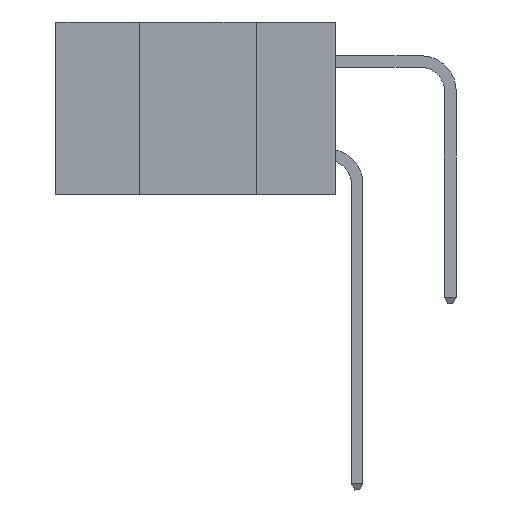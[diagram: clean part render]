
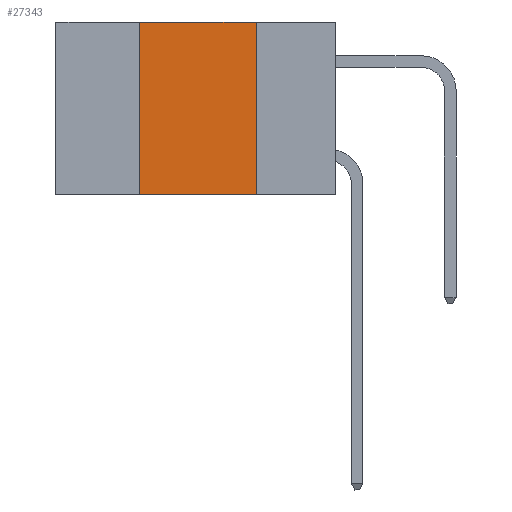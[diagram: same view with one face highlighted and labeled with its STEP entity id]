
A CAD part, left-side view. The second image highlights one B-rep face of the part: STEP entity #27343.
In plain terms, the highlighted planar face has unit normal (-1, 0, 0).
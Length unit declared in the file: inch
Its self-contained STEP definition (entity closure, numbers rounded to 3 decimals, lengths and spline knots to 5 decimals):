
#1669 = EDGE_CURVE ( 'NONE', #2630, #27662, #23827, .T. ) ;
#2630 = VERTEX_POINT ( 'NONE', #12141 ) ;
#4084 = ORIENTED_EDGE ( 'NONE', *, *, #40504, .T. ) ;
#5150 = CARTESIAN_POINT ( 'NONE',  ( 0., 0.6, -0.37 ) ) ;
#7778 = PLANE ( 'NONE',  #17568 ) ;
#11887 = CARTESIAN_POINT ( 'NONE',  ( 0., 0.42, 0. ) ) ;
#12141 = CARTESIAN_POINT ( 'NONE',  ( 0., 0.42, 0. ) ) ;
#13660 = CARTESIAN_POINT ( 'NONE',  ( 0., 0.6, 0. ) ) ;
#13869 = DIRECTION ( 'NONE',  ( 0., 0., -1. ) ) ;
#14840 = LINE ( 'NONE', #11887, #42005 ) ;
#15228 = EDGE_CURVE ( 'NONE', #17603, #2630, #14840, .T. ) ;
#16314 = LINE ( 'NONE', #5150, #26080 ) ;
#17568 = AXIS2_PLACEMENT_3D ( 'NONE', #21005, #37582, #24029 ) ;
#17603 = VERTEX_POINT ( 'NONE', #34064 ) ;
#18677 = DIRECTION ( 'NONE',  ( 0., -1., 0. ) ) ;
#21005 = CARTESIAN_POINT ( 'NONE',  ( 0., 0.6, 0. ) ) ;
#22576 = VECTOR ( 'NONE', #13869, 39.37008 ) ;
#23827 = LINE ( 'NONE', #13660, #35603 ) ;
#24029 = DIRECTION ( 'NONE',  ( 0., 0., -1. ) ) ;
#24811 = EDGE_LOOP ( 'NONE', ( #26879, #31824, #26322, #4084 ) ) ;
#26080 = VECTOR ( 'NONE', #18677, 39.37008 ) ;
#26322 = ORIENTED_EDGE ( 'NONE', *, *, #15228, .F. ) ;
#26879 = ORIENTED_EDGE ( 'NONE', *, *, #39177, .F. ) ;
#27200 = LINE ( 'NONE', #40202, #22576 ) ;
#27343 = ADVANCED_FACE ( 'NONE', ( #34318 ), #7778, .F. ) ;
#27662 = VERTEX_POINT ( 'NONE', #41746 ) ;
#28092 = DIRECTION ( 'NONE',  ( 0., 0., 1. ) ) ;
#29257 = VERTEX_POINT ( 'NONE', #30743 ) ;
#30743 = CARTESIAN_POINT ( 'NONE',  ( 0., 0.17, -0.37 ) ) ;
#31824 = ORIENTED_EDGE ( 'NONE', *, *, #1669, .F. ) ;
#34064 = CARTESIAN_POINT ( 'NONE',  ( 0., 0.42, -0.37 ) ) ;
#34318 = FACE_OUTER_BOUND ( 'NONE', #24811, .T. ) ;
#35603 = VECTOR ( 'NONE', #36547, 39.37008 ) ;
#36547 = DIRECTION ( 'NONE',  ( 0., -1., 0. ) ) ;
#37582 = DIRECTION ( 'NONE',  ( 1., 0., 0. ) ) ;
#39177 = EDGE_CURVE ( 'NONE', #27662, #29257, #27200, .T. ) ;
#40202 = CARTESIAN_POINT ( 'NONE',  ( 0., 0.17, 0. ) ) ;
#40504 = EDGE_CURVE ( 'NONE', #17603, #29257, #16314, .T. ) ;
#41746 = CARTESIAN_POINT ( 'NONE',  ( 0., 0.17, 0. ) ) ;
#42005 = VECTOR ( 'NONE', #28092, 39.37008 ) ;
